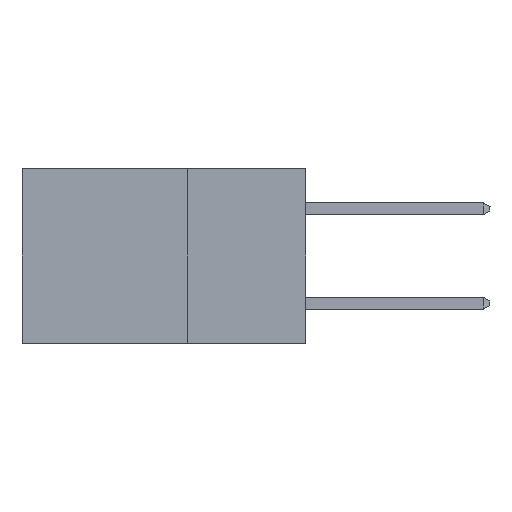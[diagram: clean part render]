
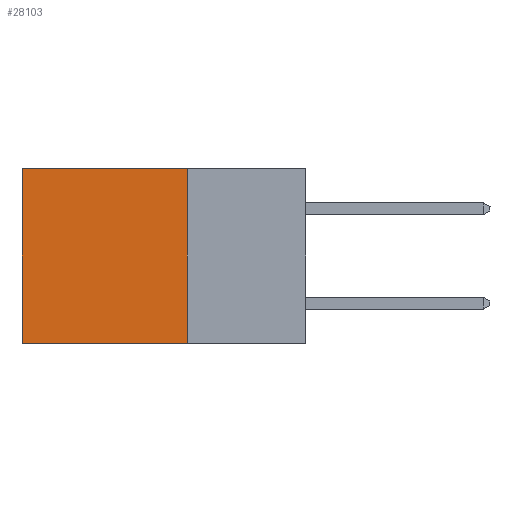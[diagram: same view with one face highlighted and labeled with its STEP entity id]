
A CAD part, left-side view. The second image highlights one B-rep face of the part: STEP entity #28103.
In plain terms, the highlighted planar face has unit normal (-1, 0, 0).
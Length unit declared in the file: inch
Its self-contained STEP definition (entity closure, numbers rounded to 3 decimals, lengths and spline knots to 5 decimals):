
#310 = LINE ( 'NONE', #18000, #26329 ) ;
#882 = VERTEX_POINT ( 'NONE', #16472 ) ;
#1482 = VERTEX_POINT ( 'NONE', #13530 ) ;
#2292 = ORIENTED_EDGE ( 'NONE', *, *, #2373, .T. ) ;
#2361 = CARTESIAN_POINT ( 'NONE',  ( 0.298, 0.25, 0. ) ) ;
#2373 = EDGE_CURVE ( 'NONE', #1482, #20685, #310, .T. ) ;
#2530 = CARTESIAN_POINT ( 'NONE',  ( 0.298, 0.25, -0.37 ) ) ;
#2605 = LINE ( 'NONE', #2530, #11673 ) ;
#3014 = DIRECTION ( 'NONE',  ( 0., 0., -1. ) ) ;
#3082 = EDGE_CURVE ( 'NONE', #882, #1482, #17148, .T. ) ;
#5498 = CARTESIAN_POINT ( 'NONE',  ( 0.298, 0.25, -0.37 ) ) ;
#7460 = DIRECTION ( 'NONE',  ( 0., 0., -1. ) ) ;
#8438 = EDGE_CURVE ( 'NONE', #12870, #20685, #2605, .T. ) ;
#9047 = LINE ( 'NONE', #29453, #17263 ) ;
#9130 = ORIENTED_EDGE ( 'NONE', *, *, #8438, .F. ) ;
#9947 = DIRECTION ( 'NONE',  ( 0., 1., 0. ) ) ;
#10165 = ORIENTED_EDGE ( 'NONE', *, *, #20262, .F. ) ;
#11086 = DIRECTION ( 'NONE',  ( 0., 1., 0. ) ) ;
#11673 = VECTOR ( 'NONE', #9947, 39.37008 ) ;
#12487 = DIRECTION ( 'NONE',  ( 0., 0., -1. ) ) ;
#12870 = VERTEX_POINT ( 'NONE', #5498 ) ;
#13530 = CARTESIAN_POINT ( 'NONE',  ( 0.298, 0.6, 0. ) ) ;
#14925 = CARTESIAN_POINT ( 'NONE',  ( 0.298, 0.6, -0.37 ) ) ;
#15885 = CARTESIAN_POINT ( 'NONE',  ( 0.298, 0.25, 0. ) ) ;
#16472 = CARTESIAN_POINT ( 'NONE',  ( 0.298, 0.25, 0. ) ) ;
#17148 = LINE ( 'NONE', #15885, #25438 ) ;
#17263 = VECTOR ( 'NONE', #12487, 39.37008 ) ;
#18000 = CARTESIAN_POINT ( 'NONE',  ( 0.298, 0.6, 0. ) ) ;
#18287 = ORIENTED_EDGE ( 'NONE', *, *, #3082, .T. ) ;
#19684 = DIRECTION ( 'NONE',  ( 1., 0., 0. ) ) ;
#20262 = EDGE_CURVE ( 'NONE', #882, #12870, #9047, .T. ) ;
#20685 = VERTEX_POINT ( 'NONE', #14925 ) ;
#25438 = VECTOR ( 'NONE', #11086, 39.37008 ) ;
#26219 = AXIS2_PLACEMENT_3D ( 'NONE', #2361, #19684, #7460 ) ;
#26329 = VECTOR ( 'NONE', #3014, 39.37008 ) ;
#27488 = EDGE_LOOP ( 'NONE', ( #2292, #9130, #10165, #18287 ) ) ;
#28103 = ADVANCED_FACE ( 'NONE', ( #32481 ), #29546, .F. ) ;
#29453 = CARTESIAN_POINT ( 'NONE',  ( 0.298, 0.25, 0. ) ) ;
#29546 = PLANE ( 'NONE',  #26219 ) ;
#32481 = FACE_OUTER_BOUND ( 'NONE', #27488, .T. ) ;
